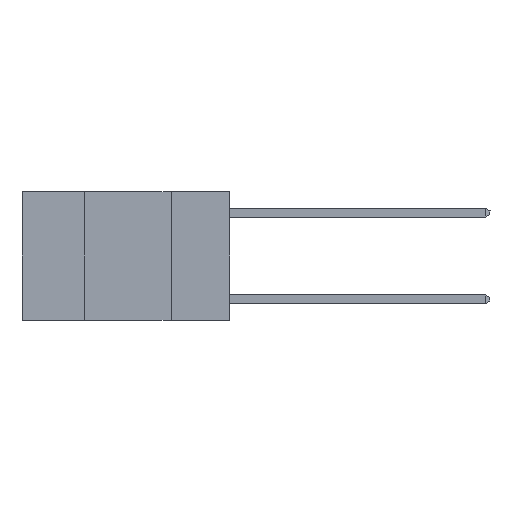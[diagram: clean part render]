
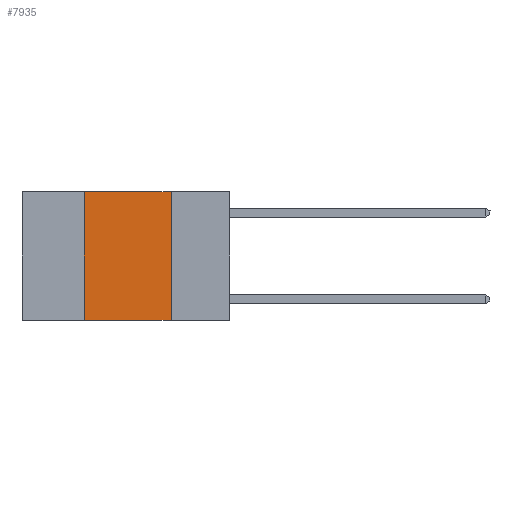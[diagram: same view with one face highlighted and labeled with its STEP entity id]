
A CAD part, left-side view. The second image highlights one B-rep face of the part: STEP entity #7935.
In plain terms, the highlighted planar face has unit normal (-1, 0, 0).
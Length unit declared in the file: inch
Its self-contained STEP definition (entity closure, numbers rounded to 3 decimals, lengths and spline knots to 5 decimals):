
#230 = ORIENTED_EDGE ( 'NONE', *, *, #14246, .F. ) ;
#381 = LINE ( 'NONE', #13836, #3238 ) ;
#693 = LINE ( 'NONE', #6052, #12828 ) ;
#874 = FACE_OUTER_BOUND ( 'NONE', #5698, .T. ) ;
#2182 = VERTEX_POINT ( 'NONE', #6900 ) ;
#2435 = DIRECTION ( 'NONE',  ( 0., 0., 1. ) ) ;
#2977 = EDGE_CURVE ( 'NONE', #11013, #11139, #6516, .T. ) ;
#3238 = VECTOR ( 'NONE', #15040, 39.37008 ) ;
#3353 = CARTESIAN_POINT ( 'NONE',  ( 0., 0.6, -0.37 ) ) ;
#4117 = DIRECTION ( 'NONE',  ( 0., 0., -1. ) ) ;
#4397 = ORIENTED_EDGE ( 'NONE', *, *, #5646, .T. ) ;
#5416 = DIRECTION ( 'NONE',  ( 0., 0., -1. ) ) ;
#5646 = EDGE_CURVE ( 'NONE', #6588, #11139, #12715, .T. ) ;
#5698 = EDGE_LOOP ( 'NONE', ( #14182, #230, #11795, #4397 ) ) ;
#6052 = CARTESIAN_POINT ( 'NONE',  ( 0., 0.42, 0. ) ) ;
#6516 = LINE ( 'NONE', #14777, #9377 ) ;
#6532 = CARTESIAN_POINT ( 'NONE',  ( 0., 0.42, -0.37 ) ) ;
#6588 = VERTEX_POINT ( 'NONE', #6532 ) ;
#6675 = AXIS2_PLACEMENT_3D ( 'NONE', #14960, #11365, #4117 ) ;
#6900 = CARTESIAN_POINT ( 'NONE',  ( 0., 0.42, 0. ) ) ;
#7935 = ADVANCED_FACE ( 'NONE', ( #874 ), #8941, .F. ) ;
#8941 = PLANE ( 'NONE',  #6675 ) ;
#9377 = VECTOR ( 'NONE', #5416, 39.37008 ) ;
#9635 = EDGE_CURVE ( 'NONE', #6588, #2182, #693, .T. ) ;
#9878 = VECTOR ( 'NONE', #13028, 39.37008 ) ;
#9935 = CARTESIAN_POINT ( 'NONE',  ( 0., 0.17, -0.37 ) ) ;
#11013 = VERTEX_POINT ( 'NONE', #14529 ) ;
#11139 = VERTEX_POINT ( 'NONE', #9935 ) ;
#11365 = DIRECTION ( 'NONE',  ( 1., 0., 0. ) ) ;
#11795 = ORIENTED_EDGE ( 'NONE', *, *, #9635, .F. ) ;
#12715 = LINE ( 'NONE', #3353, #9878 ) ;
#12828 = VECTOR ( 'NONE', #2435, 39.37008 ) ;
#13028 = DIRECTION ( 'NONE',  ( 0., -1., 0. ) ) ;
#13836 = CARTESIAN_POINT ( 'NONE',  ( 0., 0.6, 0. ) ) ;
#14182 = ORIENTED_EDGE ( 'NONE', *, *, #2977, .F. ) ;
#14246 = EDGE_CURVE ( 'NONE', #2182, #11013, #381, .T. ) ;
#14529 = CARTESIAN_POINT ( 'NONE',  ( 0., 0.17, 0. ) ) ;
#14777 = CARTESIAN_POINT ( 'NONE',  ( 0., 0.17, 0. ) ) ;
#14960 = CARTESIAN_POINT ( 'NONE',  ( 0., 0.6, 0. ) ) ;
#15040 = DIRECTION ( 'NONE',  ( 0., -1., 0. ) ) ;
